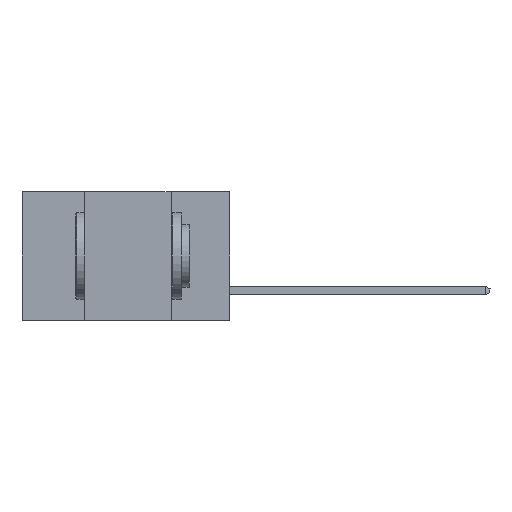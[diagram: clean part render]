
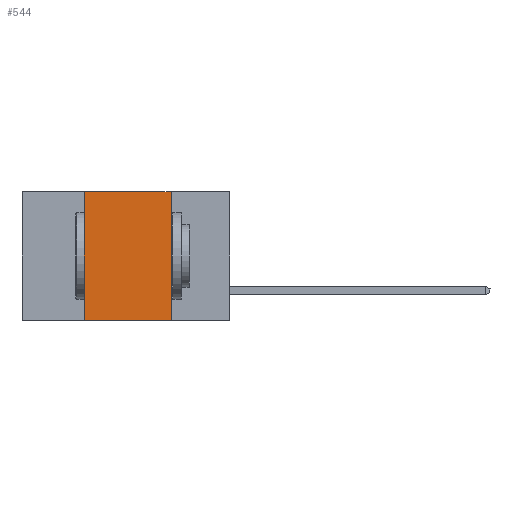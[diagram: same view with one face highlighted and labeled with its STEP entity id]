
A CAD part, left-side view. The second image highlights one B-rep face of the part: STEP entity #544.
In plain terms, the highlighted planar face has unit normal (-1, 0, 0).
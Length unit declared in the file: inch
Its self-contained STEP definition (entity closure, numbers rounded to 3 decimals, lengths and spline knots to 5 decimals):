
#300 = VERTEX_POINT ( 'NONE', #959 ) ;
#342 = CARTESIAN_POINT ( 'NONE',  ( 0., 0.42, -0.37 ) ) ;
#383 = VERTEX_POINT ( 'NONE', #342 ) ;
#544 = ADVANCED_FACE ( 'NONE', ( #8294 ), #6657, .F. ) ;
#556 = DIRECTION ( 'NONE',  ( 1., 0., 0. ) ) ;
#576 = LINE ( 'NONE', #10104, #7753 ) ;
#608 = CARTESIAN_POINT ( 'NONE',  ( 0., 0.6, 0. ) ) ;
#645 = VECTOR ( 'NONE', #766, 39.37008 ) ;
#766 = DIRECTION ( 'NONE',  ( 0., -1., 0. ) ) ;
#959 = CARTESIAN_POINT ( 'NONE',  ( 0., 0.42, 0. ) ) ;
#988 = VECTOR ( 'NONE', #4129, 39.37008 ) ;
#1019 = EDGE_CURVE ( 'NONE', #383, #300, #9564, .T. ) ;
#1289 = CARTESIAN_POINT ( 'NONE',  ( 0., 0.17, -0.37 ) ) ;
#1548 = LINE ( 'NONE', #10236, #645 ) ;
#1840 = ORIENTED_EDGE ( 'NONE', *, *, #6906, .T. ) ;
#2073 = EDGE_LOOP ( 'NONE', ( #7859, #4412, #8642, #1840 ) ) ;
#2275 = CARTESIAN_POINT ( 'NONE',  ( 0., 0.17, 0. ) ) ;
#2976 = VERTEX_POINT ( 'NONE', #1289 ) ;
#3551 = AXIS2_PLACEMENT_3D ( 'NONE', #608, #556, #8352 ) ;
#4129 = DIRECTION ( 'NONE',  ( 0., -1., 0. ) ) ;
#4340 = CARTESIAN_POINT ( 'NONE',  ( 0., 0.42, -0.37 ) ) ;
#4412 = ORIENTED_EDGE ( 'NONE', *, *, #10912, .F. ) ;
#4936 = DIRECTION ( 'NONE',  ( 0., 0., -1. ) ) ;
#4964 = LINE ( 'NONE', #10134, #988 ) ;
#6657 = PLANE ( 'NONE',  #3551 ) ;
#6906 = EDGE_CURVE ( 'NONE', #383, #2976, #4964, .T. ) ;
#6974 = VECTOR ( 'NONE', #10227, 39.37008 ) ;
#7694 = EDGE_CURVE ( 'NONE', #9362, #2976, #576, .T. ) ;
#7753 = VECTOR ( 'NONE', #4936, 39.37008 ) ;
#7859 = ORIENTED_EDGE ( 'NONE', *, *, #7694, .F. ) ;
#8294 = FACE_OUTER_BOUND ( 'NONE', #2073, .T. ) ;
#8352 = DIRECTION ( 'NONE',  ( 0., 0., -1. ) ) ;
#8642 = ORIENTED_EDGE ( 'NONE', *, *, #1019, .F. ) ;
#9362 = VERTEX_POINT ( 'NONE', #2275 ) ;
#9564 = LINE ( 'NONE', #4340, #6974 ) ;
#10104 = CARTESIAN_POINT ( 'NONE',  ( 0., 0.17, -0.37 ) ) ;
#10134 = CARTESIAN_POINT ( 'NONE',  ( 0., 0.6, -0.37 ) ) ;
#10227 = DIRECTION ( 'NONE',  ( 0., 0., 1. ) ) ;
#10236 = CARTESIAN_POINT ( 'NONE',  ( 0., 0.6, 0. ) ) ;
#10912 = EDGE_CURVE ( 'NONE', #300, #9362, #1548, .T. ) ;
